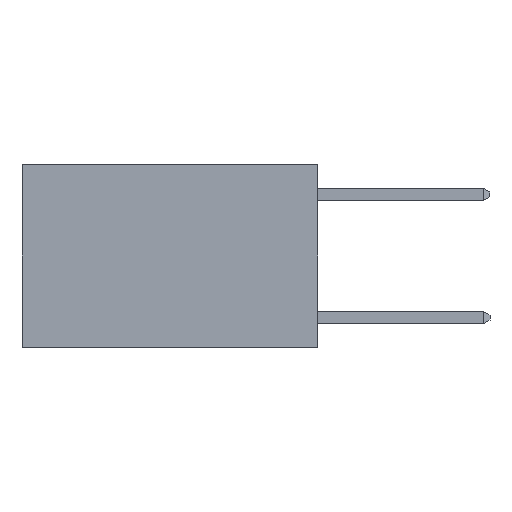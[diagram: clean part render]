
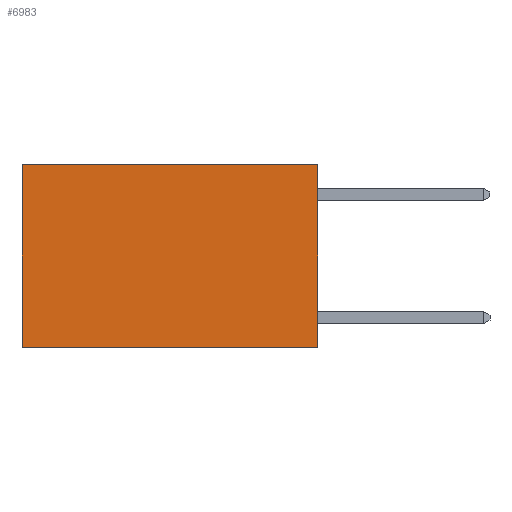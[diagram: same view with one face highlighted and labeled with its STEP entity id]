
A CAD part, left-side view. The second image highlights one B-rep face of the part: STEP entity #6983.
In plain terms, the highlighted planar face has unit normal (-1, 0, 0).
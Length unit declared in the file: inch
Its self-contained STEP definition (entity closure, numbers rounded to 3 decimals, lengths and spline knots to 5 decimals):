
#477 = EDGE_CURVE ( 'NONE', #4420, #7464, #8004, .T. ) ;
#522 = CARTESIAN_POINT ( 'NONE',  ( 0.2625, 0.6, -0.37 ) ) ;
#713 = DIRECTION ( 'NONE',  ( 0., 1., 0. ) ) ;
#961 = FACE_OUTER_BOUND ( 'NONE', #5766, .T. ) ;
#2498 = DIRECTION ( 'NONE',  ( 0., 0., -1. ) ) ;
#2555 = VECTOR ( 'NONE', #3336, 39.37008 ) ;
#2558 = CARTESIAN_POINT ( 'NONE',  ( 0.2625, 0., 0. ) ) ;
#2860 = ORIENTED_EDGE ( 'NONE', *, *, #9235, .T. ) ;
#3336 = DIRECTION ( 'NONE',  ( 0., 0., -1. ) ) ;
#3753 = VECTOR ( 'NONE', #6681, 39.37008 ) ;
#3836 = ORIENTED_EDGE ( 'NONE', *, *, #477, .T. ) ;
#4196 = EDGE_CURVE ( 'NONE', #5698, #10100, #6199, .T. ) ;
#4239 = VECTOR ( 'NONE', #2498, 39.37008 ) ;
#4332 = CARTESIAN_POINT ( 'NONE',  ( 0.2625, 0., 0. ) ) ;
#4393 = EDGE_CURVE ( 'NONE', #4420, #5698, #8467, .T. ) ;
#4420 = VERTEX_POINT ( 'NONE', #2558 ) ;
#4868 = AXIS2_PLACEMENT_3D ( 'NONE', #4332, #9872, #5137 ) ;
#5137 = DIRECTION ( 'NONE',  ( 0., 0., -1. ) ) ;
#5698 = VERTEX_POINT ( 'NONE', #8897 ) ;
#5766 = EDGE_LOOP ( 'NONE', ( #2860, #10292, #10145, #3836 ) ) ;
#6199 = LINE ( 'NONE', #10201, #10190 ) ;
#6422 = CARTESIAN_POINT ( 'NONE',  ( 0.2625, 0.6, 0. ) ) ;
#6645 = PLANE ( 'NONE',  #4868 ) ;
#6681 = DIRECTION ( 'NONE',  ( 0., 1., 0. ) ) ;
#6707 = CARTESIAN_POINT ( 'NONE',  ( 0.2625, 0., 0. ) ) ;
#6778 = LINE ( 'NONE', #8116, #2555 ) ;
#6983 = ADVANCED_FACE ( 'NONE', ( #961 ), #6645, .F. ) ;
#7464 = VERTEX_POINT ( 'NONE', #6422 ) ;
#8004 = LINE ( 'NONE', #6707, #3753 ) ;
#8060 = CARTESIAN_POINT ( 'NONE',  ( 0.2625, 0., 0. ) ) ;
#8116 = CARTESIAN_POINT ( 'NONE',  ( 0.2625, 0.6, 0. ) ) ;
#8467 = LINE ( 'NONE', #8060, #4239 ) ;
#8897 = CARTESIAN_POINT ( 'NONE',  ( 0.2625, 0., -0.37 ) ) ;
#9235 = EDGE_CURVE ( 'NONE', #7464, #10100, #6778, .T. ) ;
#9872 = DIRECTION ( 'NONE',  ( 1., 0., 0. ) ) ;
#10100 = VERTEX_POINT ( 'NONE', #522 ) ;
#10145 = ORIENTED_EDGE ( 'NONE', *, *, #4393, .F. ) ;
#10190 = VECTOR ( 'NONE', #713, 39.37008 ) ;
#10201 = CARTESIAN_POINT ( 'NONE',  ( 0.2625, 0., -0.37 ) ) ;
#10292 = ORIENTED_EDGE ( 'NONE', *, *, #4196, .F. ) ;
